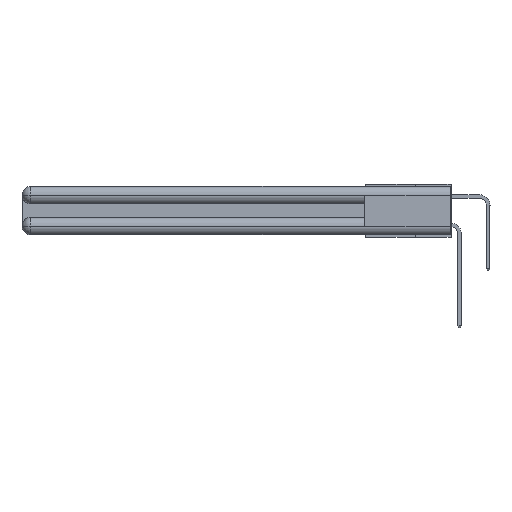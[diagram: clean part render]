
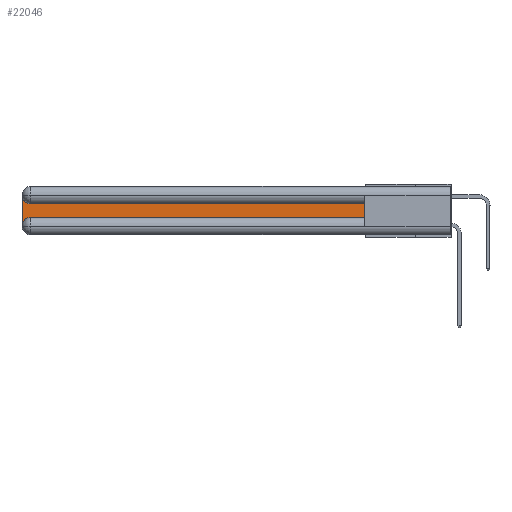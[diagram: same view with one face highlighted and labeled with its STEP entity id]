
A CAD part, left-side view. The second image highlights one B-rep face of the part: STEP entity #22046.
In plain terms, the highlighted planar face has unit normal (-1, 0, 0).
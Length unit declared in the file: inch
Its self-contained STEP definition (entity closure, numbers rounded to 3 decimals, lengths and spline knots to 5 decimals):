
#162 = ORIENTED_EDGE ( 'NONE', *, *, #22053, .T. ) ;
#696 = EDGE_CURVE ( 'NONE', #6221, #28396, #8638, .T. ) ;
#838 = DIRECTION ( 'NONE',  ( 0., 0., -1. ) ) ;
#1324 = VERTEX_POINT ( 'NONE', #11136 ) ;
#2034 = CIRCLE ( 'NONE', #2771, 0.06 ) ;
#2367 = VECTOR ( 'NONE', #2852, 39.37008 ) ;
#2771 = AXIS2_PLACEMENT_3D ( 'NONE', #12138, #25678, #12045 ) ;
#2852 = DIRECTION ( 'NONE',  ( 0., 1., 0. ) ) ;
#4023 = ORIENTED_EDGE ( 'NONE', *, *, #25572, .T. ) ;
#4156 = DIRECTION ( 'NONE',  ( 0., -1., 0. ) ) ;
#6038 = CARTESIAN_POINT ( 'NONE',  ( 0.075, 3., -0.2775 ) ) ;
#6221 = VERTEX_POINT ( 'NONE', #15306 ) ;
#7064 = VECTOR ( 'NONE', #24614, 39.37008 ) ;
#7187 = VERTEX_POINT ( 'NONE', #8959 ) ;
#7334 = DIRECTION ( 'NONE',  ( 1., 0., 0. ) ) ;
#8448 = CARTESIAN_POINT ( 'NONE',  ( 0.075, 3., -0.2175 ) ) ;
#8615 = AXIS2_PLACEMENT_3D ( 'NONE', #21543, #9761, #838 ) ;
#8638 = LINE ( 'NONE', #29383, #18465 ) ;
#8959 = CARTESIAN_POINT ( 'NONE',  ( 0.075, 3., -0.0625 ) ) ;
#9448 = DIRECTION ( 'NONE',  ( 0., 0., -1. ) ) ;
#9761 = DIRECTION ( 'NONE',  ( 1., 0., 0. ) ) ;
#11136 = CARTESIAN_POINT ( 'NONE',  ( 0.075, 0.6, -0.1225 ) ) ;
#11168 = CARTESIAN_POINT ( 'NONE',  ( 0.075, 0.6, -0.2175 ) ) ;
#12045 = DIRECTION ( 'NONE',  ( 0., 0., -1. ) ) ;
#12138 = CARTESIAN_POINT ( 'NONE',  ( 0.075, 2.94, -0.0625 ) ) ;
#12176 = EDGE_CURVE ( 'NONE', #7187, #16937, #13171, .T. ) ;
#12216 = ORIENTED_EDGE ( 'NONE', *, *, #27828, .T. ) ;
#13171 = LINE ( 'NONE', #8448, #7064 ) ;
#14762 = ORIENTED_EDGE ( 'NONE', *, *, #22090, .T. ) ;
#15306 = CARTESIAN_POINT ( 'NONE',  ( 0.075, 2.94, -0.2175 ) ) ;
#15319 = ORIENTED_EDGE ( 'NONE', *, *, #12176, .T. ) ;
#16866 = PLANE ( 'NONE',  #8615 ) ;
#16937 = VERTEX_POINT ( 'NONE', #6038 ) ;
#18258 = LINE ( 'NONE', #25936, #2367 ) ;
#18465 = VECTOR ( 'NONE', #4156, 39.37008 ) ;
#20008 = ORIENTED_EDGE ( 'NONE', *, *, #696, .T. ) ;
#20444 = VECTOR ( 'NONE', #24802, 39.37008 ) ;
#21543 = CARTESIAN_POINT ( 'NONE',  ( 0.075, 3., -0.1225 ) ) ;
#21892 = FACE_OUTER_BOUND ( 'NONE', #23344, .T. ) ;
#22046 = ADVANCED_FACE ( 'NONE', ( #21892 ), #16866, .F. ) ;
#22053 = EDGE_CURVE ( 'NONE', #1324, #28654, #18258, .T. ) ;
#22090 = EDGE_CURVE ( 'NONE', #28396, #1324, #26858, .T. ) ;
#22206 = CARTESIAN_POINT ( 'NONE',  ( 0.075, 2.94, -0.1225 ) ) ;
#23344 = EDGE_LOOP ( 'NONE', ( #162, #4023, #15319, #12216, #20008, #14762 ) ) ;
#23505 = CARTESIAN_POINT ( 'NONE',  ( 0.075, 2.94, -0.2775 ) ) ;
#24614 = DIRECTION ( 'NONE',  ( 0., 0., -1. ) ) ;
#24802 = DIRECTION ( 'NONE',  ( 0., 0., 1. ) ) ;
#24946 = CIRCLE ( 'NONE', #29627, 0.06 ) ;
#25572 = EDGE_CURVE ( 'NONE', #28654, #7187, #2034, .T. ) ;
#25678 = DIRECTION ( 'NONE',  ( 1., 0., 0. ) ) ;
#25936 = CARTESIAN_POINT ( 'NONE',  ( 0.075, 0.6, -0.1225 ) ) ;
#26858 = LINE ( 'NONE', #26888, #20444 ) ;
#26888 = CARTESIAN_POINT ( 'NONE',  ( 0.075, 0.6, -0.2175 ) ) ;
#27828 = EDGE_CURVE ( 'NONE', #16937, #6221, #24946, .T. ) ;
#28396 = VERTEX_POINT ( 'NONE', #11168 ) ;
#28654 = VERTEX_POINT ( 'NONE', #22206 ) ;
#29383 = CARTESIAN_POINT ( 'NONE',  ( 0.075, 0.6, -0.2175 ) ) ;
#29627 = AXIS2_PLACEMENT_3D ( 'NONE', #23505, #7334, #9448 ) ;
